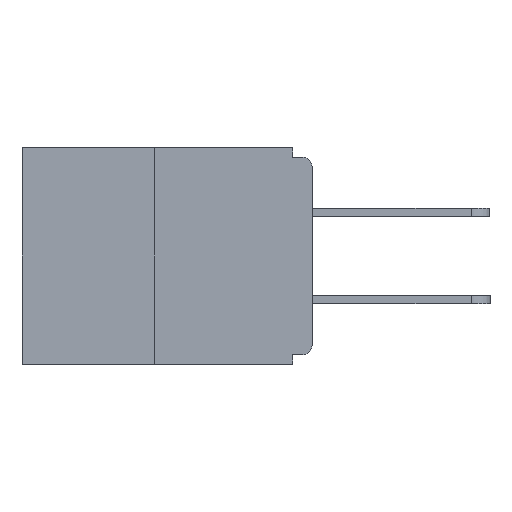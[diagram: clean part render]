
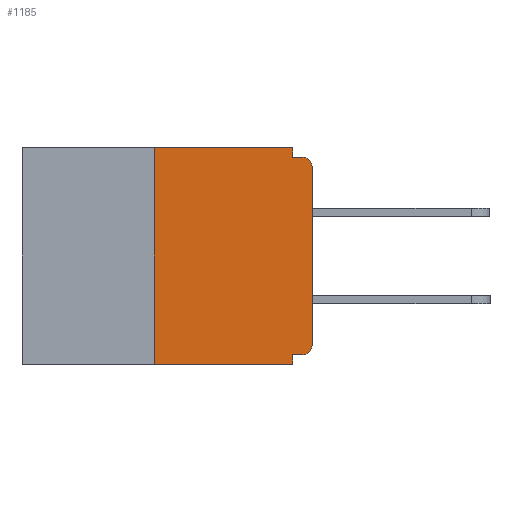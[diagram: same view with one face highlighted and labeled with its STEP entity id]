
A CAD part, left-side view. The second image highlights one B-rep face of the part: STEP entity #1185.
In plain terms, the highlighted planar face has unit normal (-1, 0, 0).
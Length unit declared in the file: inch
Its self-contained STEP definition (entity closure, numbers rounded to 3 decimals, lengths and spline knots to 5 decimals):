
#33 = PLANE ( 'NONE',  #19528 ) ;
#111 = CARTESIAN_POINT ( 'NONE',  ( 0., 0.46, 0. ) ) ;
#574 = VERTEX_POINT ( 'NONE', #22243 ) ;
#588 = ORIENTED_EDGE ( 'NONE', *, *, #20932, .F. ) ;
#985 = LINE ( 'NONE', #20793, #1308 ) ;
#1185 = ADVANCED_FACE ( 'NONE', ( #17387 ), #33, .F. ) ;
#1308 = VECTOR ( 'NONE', #13599, 39.37008 ) ;
#2050 = CIRCLE ( 'NONE', #7884, 0.015 ) ;
#2444 = EDGE_CURVE ( 'NONE', #9217, #3724, #2050, .T. ) ;
#2839 = DIRECTION ( 'NONE',  ( 0., -1., 0. ) ) ;
#3042 = CARTESIAN_POINT ( 'NONE',  ( 0., 0.031, 0. ) ) ;
#3145 = DIRECTION ( 'NONE',  ( 0., 0., 1. ) ) ;
#3155 = VECTOR ( 'NONE', #3145, 39.37008 ) ;
#3724 = VERTEX_POINT ( 'NONE', #13619 ) ;
#3733 = CARTESIAN_POINT ( 'NONE',  ( 0., 0., -0.313 ) ) ;
#3819 = CARTESIAN_POINT ( 'NONE',  ( 0., 0.031, 0. ) ) ;
#3823 = CARTESIAN_POINT ( 'NONE',  ( 0., 0.015, -0.03 ) ) ;
#4015 = VECTOR ( 'NONE', #7873, 39.37008 ) ;
#4465 = ORIENTED_EDGE ( 'NONE', *, *, #8063, .T. ) ;
#5164 = VECTOR ( 'NONE', #2839, 39.37008 ) ;
#5826 = DIRECTION ( 'NONE',  ( 0., 0., -1. ) ) ;
#5888 = VERTEX_POINT ( 'NONE', #22614 ) ;
#5954 = EDGE_CURVE ( 'NONE', #574, #5888, #14434, .T. ) ;
#6372 = VECTOR ( 'NONE', #11884, 39.37008 ) ;
#6760 = DIRECTION ( 'NONE',  ( 0., 0., 1. ) ) ;
#7085 = CARTESIAN_POINT ( 'NONE',  ( 0., 0., -0.03 ) ) ;
#7165 = DIRECTION ( 'NONE',  ( -1., 0., 0. ) ) ;
#7644 = LINE ( 'NONE', #3819, #15999 ) ;
#7873 = DIRECTION ( 'NONE',  ( 0., 1., 0. ) ) ;
#7884 = AXIS2_PLACEMENT_3D ( 'NONE', #3823, #7165, #14723 ) ;
#7992 = EDGE_CURVE ( 'NONE', #9573, #20891, #16809, .T. ) ;
#8063 = EDGE_CURVE ( 'NONE', #9775, #14950, #18099, .T. ) ;
#8224 = ORIENTED_EDGE ( 'NONE', *, *, #23334, .F. ) ;
#8264 = ORIENTED_EDGE ( 'NONE', *, *, #7992, .F. ) ;
#8297 = ORIENTED_EDGE ( 'NONE', *, *, #2444, .T. ) ;
#8509 = CARTESIAN_POINT ( 'NONE',  ( 0., 0., 0. ) ) ;
#8551 = ORIENTED_EDGE ( 'NONE', *, *, #14296, .F. ) ;
#9217 = VERTEX_POINT ( 'NONE', #7085 ) ;
#9381 = CARTESIAN_POINT ( 'NONE',  ( 0., 0., -0.015 ) ) ;
#9573 = VERTEX_POINT ( 'NONE', #17542 ) ;
#9601 = CARTESIAN_POINT ( 'NONE',  ( 0., 0.015, -0.328 ) ) ;
#9775 = VERTEX_POINT ( 'NONE', #9601 ) ;
#10342 = LINE ( 'NONE', #8509, #18692 ) ;
#11554 = AXIS2_PLACEMENT_3D ( 'NONE', #16710, #18595, #12854 ) ;
#11865 = DIRECTION ( 'NONE',  ( 0., 0., -1. ) ) ;
#11884 = DIRECTION ( 'NONE',  ( 0., 0., -1. ) ) ;
#11927 = LINE ( 'NONE', #9381, #20012 ) ;
#12033 = LINE ( 'NONE', #20990, #4015 ) ;
#12106 = LINE ( 'NONE', #24041, #3155 ) ;
#12573 = ORIENTED_EDGE ( 'NONE', *, *, #5954, .F. ) ;
#12854 = DIRECTION ( 'NONE',  ( 0., 0., -1. ) ) ;
#13599 = DIRECTION ( 'NONE',  ( 0., -1., 0. ) ) ;
#13619 = CARTESIAN_POINT ( 'NONE',  ( 0., 0.015, -0.015 ) ) ;
#13799 = VERTEX_POINT ( 'NONE', #18256 ) ;
#14094 = CARTESIAN_POINT ( 'NONE',  ( 0., 0.031, -0.015 ) ) ;
#14296 = EDGE_CURVE ( 'NONE', #9775, #574, #12033, .T. ) ;
#14434 = LINE ( 'NONE', #21266, #6372 ) ;
#14723 = DIRECTION ( 'NONE',  ( 0., 0., -1. ) ) ;
#14873 = DIRECTION ( 'NONE',  ( 0., -1., 0. ) ) ;
#14950 = VERTEX_POINT ( 'NONE', #3733 ) ;
#15546 = DIRECTION ( 'NONE',  ( 1., 0., 0. ) ) ;
#15679 = VERTEX_POINT ( 'NONE', #14094 ) ;
#15999 = VECTOR ( 'NONE', #5826, 39.37008 ) ;
#16710 = CARTESIAN_POINT ( 'NONE',  ( 0., 0.015, -0.313 ) ) ;
#16809 = LINE ( 'NONE', #18086, #5164 ) ;
#17387 = FACE_OUTER_BOUND ( 'NONE', #18346, .T. ) ;
#17542 = CARTESIAN_POINT ( 'NONE',  ( 0., 0.25, 0. ) ) ;
#18086 = CARTESIAN_POINT ( 'NONE',  ( 0., 0.46, 0. ) ) ;
#18099 = CIRCLE ( 'NONE', #11554, 0.015 ) ;
#18250 = ORIENTED_EDGE ( 'NONE', *, *, #18411, .T. ) ;
#18256 = CARTESIAN_POINT ( 'NONE',  ( 0., 0.25, -0.343 ) ) ;
#18346 = EDGE_LOOP ( 'NONE', ( #8264, #8224, #21854, #12573, #8551, #4465, #18250, #8297, #588, #20829 ) ) ;
#18411 = EDGE_CURVE ( 'NONE', #14950, #9217, #10342, .T. ) ;
#18595 = DIRECTION ( 'NONE',  ( -1., 0., 0. ) ) ;
#18692 = VECTOR ( 'NONE', #6760, 39.37008 ) ;
#19528 = AXIS2_PLACEMENT_3D ( 'NONE', #111, #15546, #11865 ) ;
#20012 = VECTOR ( 'NONE', #14873, 39.37008 ) ;
#20425 = EDGE_CURVE ( 'NONE', #20891, #15679, #7644, .T. ) ;
#20793 = CARTESIAN_POINT ( 'NONE',  ( 0., 0.46, -0.343 ) ) ;
#20829 = ORIENTED_EDGE ( 'NONE', *, *, #20425, .F. ) ;
#20891 = VERTEX_POINT ( 'NONE', #3042 ) ;
#20932 = EDGE_CURVE ( 'NONE', #15679, #3724, #11927, .T. ) ;
#20990 = CARTESIAN_POINT ( 'NONE',  ( 0., 0., -0.328 ) ) ;
#21266 = CARTESIAN_POINT ( 'NONE',  ( 0., 0.031, -0.343 ) ) ;
#21854 = ORIENTED_EDGE ( 'NONE', *, *, #24032, .T. ) ;
#22243 = CARTESIAN_POINT ( 'NONE',  ( 0., 0.031, -0.328 ) ) ;
#22614 = CARTESIAN_POINT ( 'NONE',  ( 0., 0.031, -0.343 ) ) ;
#23334 = EDGE_CURVE ( 'NONE', #13799, #9573, #12106, .T. ) ;
#24032 = EDGE_CURVE ( 'NONE', #13799, #5888, #985, .T. ) ;
#24041 = CARTESIAN_POINT ( 'NONE',  ( 0., 0.25, 0. ) ) ;
